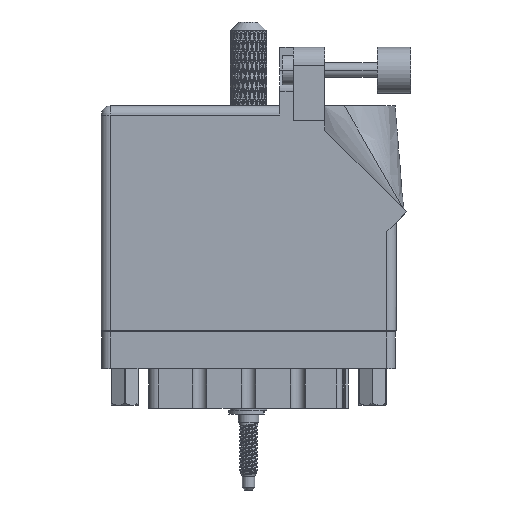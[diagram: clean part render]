
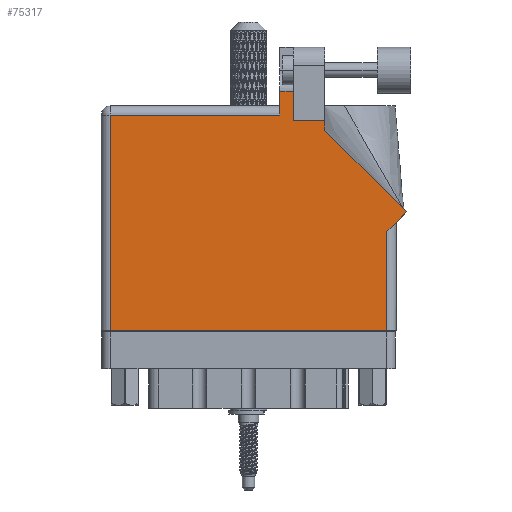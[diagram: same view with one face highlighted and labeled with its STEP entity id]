
A CAD part, front view. The second image highlights one B-rep face of the part: STEP entity #75317.
In plain terms, the highlighted face is planar.
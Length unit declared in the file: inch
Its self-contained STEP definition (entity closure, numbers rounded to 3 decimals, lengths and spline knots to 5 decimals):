
#374 = EDGE_CURVE ( 'NONE', #49870, #22491, #19610, .T. ) ;
#800 = VERTEX_POINT ( 'NONE', #60973 ) ;
#1143 = VECTOR ( 'NONE', #28978, 39.37008 ) ;
#1343 = CARTESIAN_POINT ( 'NONE',  ( 0.062, 0., 0. ) ) ;
#2345 = LINE ( 'NONE', #21454, #79653 ) ;
#4068 = CARTESIAN_POINT ( 'NONE',  ( 2.01, 0.737, 0. ) ) ;
#5318 = EDGE_CURVE ( 'NONE', #39383, #42970, #53773, .T. ) ;
#5324 = VECTOR ( 'NONE', #37915, 39.37008 ) ;
#5744 = EDGE_LOOP ( 'NONE', ( #24149, #11952, #10577, #45719, #68616, #12436, #71256, #103133, #88107, #72380, #15375 ) ) ;
#5793 = EDGE_CURVE ( 'NONE', #79085, #9011, #2345, .T. ) ;
#8879 = VECTOR ( 'NONE', #9280, 39.37008 ) ;
#9011 = VERTEX_POINT ( 'NONE', #25534 ) ;
#9280 = DIRECTION ( 'NONE',  ( -1., 0., 0. ) ) ;
#10577 = ORIENTED_EDGE ( 'NONE', *, *, #5793, .T. ) ;
#10686 = DIRECTION ( 'NONE',  ( 1., 0., 0. ) ) ;
#11869 = VECTOR ( 'NONE', #85549, 39.37008 ) ;
#11952 = ORIENTED_EDGE ( 'NONE', *, *, #102601, .T. ) ;
#12096 = CARTESIAN_POINT ( 'NONE',  ( 1.524, 1.36442, 0. ) ) ;
#12436 = ORIENTED_EDGE ( 'NONE', *, *, #32887, .T. ) ;
#14048 = DIRECTION ( 'NONE',  ( -1., 0., 0. ) ) ;
#15375 = ORIENTED_EDGE ( 'NONE', *, *, #78607, .T. ) ;
#15403 = EDGE_CURVE ( 'NONE', #61928, #29039, #55315, .T. ) ;
#19053 = CARTESIAN_POINT ( 'NONE',  ( 1.524, 1.43, 0. ) ) ;
#19610 = LINE ( 'NONE', #12096, #31677 ) ;
#21454 = CARTESIAN_POINT ( 'NONE',  ( 1.217, 1.53, 0. ) ) ;
#21537 = CARTESIAN_POINT ( 'NONE',  ( 1.311, 1.43, 0. ) ) ;
#22491 = VERTEX_POINT ( 'NONE', #109460 ) ;
#24149 = ORIENTED_EDGE ( 'NONE', *, *, #5318, .T. ) ;
#24652 = LINE ( 'NONE', #53649, #103189 ) ;
#25534 = CARTESIAN_POINT ( 'NONE',  ( 1.217, 1.468, 0. ) ) ;
#26724 = LINE ( 'NONE', #102984, #11869 ) ;
#27309 = EDGE_CURVE ( 'NONE', #29039, #800, #70169, .T. ) ;
#27651 = CARTESIAN_POINT ( 'NONE',  ( 0., 0., 0. ) ) ;
#28978 = DIRECTION ( 'NONE',  ( 0.707, 0.707, 0. ) ) ;
#29039 = VERTEX_POINT ( 'NONE', #96238 ) ;
#29055 = VERTEX_POINT ( 'NONE', #1343 ) ;
#30135 = CARTESIAN_POINT ( 'NONE',  ( 1.948, 0., 0. ) ) ;
#30700 = VECTOR ( 'NONE', #32224, 39.37008 ) ;
#31677 = VECTOR ( 'NONE', #89605, 39.37008 ) ;
#32224 = DIRECTION ( 'NONE',  ( 0., 1., 0. ) ) ;
#32887 = EDGE_CURVE ( 'NONE', #29055, #61928, #50562, .T. ) ;
#33662 = CARTESIAN_POINT ( 'NONE',  ( 0.062, 1.468, 0. ) ) ;
#37915 = DIRECTION ( 'NONE',  ( 0., 1., 0. ) ) ;
#38689 = EDGE_CURVE ( 'NONE', #46839, #29055, #26724, .T. ) ;
#39383 = VERTEX_POINT ( 'NONE', #21537 ) ;
#42509 = CARTESIAN_POINT ( 'NONE',  ( 1.948, 0.737, 0. ) ) ;
#42970 = VERTEX_POINT ( 'NONE', #43182 ) ;
#43058 = VECTOR ( 'NONE', #102209, 39.37008 ) ;
#43182 = CARTESIAN_POINT ( 'NONE',  ( 1.311, 1.6315, 0. ) ) ;
#45719 = ORIENTED_EDGE ( 'NONE', *, *, #107724, .T. ) ;
#46839 = VERTEX_POINT ( 'NONE', #33662 ) ;
#48945 = VECTOR ( 'NONE', #61003, 39.37008 ) ;
#49870 = VERTEX_POINT ( 'NONE', #84795 ) ;
#50562 = LINE ( 'NONE', #27651, #68102 ) ;
#52519 = EDGE_CURVE ( 'NONE', #800, #49870, #62511, .T. ) ;
#53649 = CARTESIAN_POINT ( 'NONE',  ( 1.64177, 1.6315, 0. ) ) ;
#53773 = LINE ( 'NONE', #83693, #30700 ) ;
#55315 = LINE ( 'NONE', #42509, #5324 ) ;
#57174 = CARTESIAN_POINT ( 'NONE',  ( 0., 1.53, 0. ) ) ;
#57375 = AXIS2_PLACEMENT_3D ( 'NONE', #57174, #91932, #14048 ) ;
#57418 = DIRECTION ( 'NONE',  ( 0., -1., 0. ) ) ;
#60973 = CARTESIAN_POINT ( 'NONE',  ( 2.08071, 0.80771, 0. ) ) ;
#61003 = DIRECTION ( 'NONE',  ( -0.707, 0.707, 0. ) ) ;
#61928 = VERTEX_POINT ( 'NONE', #30135 ) ;
#62511 = LINE ( 'NONE', #86646, #48945 ) ;
#66262 = CARTESIAN_POINT ( 'NONE',  ( 0., 1.468, 0. ) ) ;
#66988 = LINE ( 'NONE', #19053, #8879 ) ;
#68102 = VECTOR ( 'NONE', #10686, 39.37008 ) ;
#68616 = ORIENTED_EDGE ( 'NONE', *, *, #38689, .T. ) ;
#70169 = LINE ( 'NONE', #4068, #1143 ) ;
#70696 = DIRECTION ( 'NONE',  ( -1., 0., 0. ) ) ;
#71099 = CARTESIAN_POINT ( 'NONE',  ( 1.217, 1.6315, 0. ) ) ;
#71256 = ORIENTED_EDGE ( 'NONE', *, *, #15403, .T. ) ;
#72380 = ORIENTED_EDGE ( 'NONE', *, *, #374, .T. ) ;
#75317 = ADVANCED_FACE ( 'NONE', ( #77226 ), #101438, .F. ) ;
#77226 = FACE_OUTER_BOUND ( 'NONE', #5744, .T. ) ;
#78607 = EDGE_CURVE ( 'NONE', #22491, #39383, #66988, .T. ) ;
#79085 = VERTEX_POINT ( 'NONE', #71099 ) ;
#79653 = VECTOR ( 'NONE', #57418, 39.37008 ) ;
#83693 = CARTESIAN_POINT ( 'NONE',  ( 1.311, 1.43, 0. ) ) ;
#84795 = CARTESIAN_POINT ( 'NONE',  ( 1.524, 1.36442, 0. ) ) ;
#85549 = DIRECTION ( 'NONE',  ( 0., -1., 0. ) ) ;
#86646 = CARTESIAN_POINT ( 'NONE',  ( 2.08071, 0.80771, 0. ) ) ;
#88107 = ORIENTED_EDGE ( 'NONE', *, *, #52519, .T. ) ;
#89605 = DIRECTION ( 'NONE',  ( 0., 1., 0. ) ) ;
#91932 = DIRECTION ( 'NONE',  ( 0., 0., -1. ) ) ;
#96238 = CARTESIAN_POINT ( 'NONE',  ( 1.948, 0.675, 0. ) ) ;
#98543 = LINE ( 'NONE', #66262, #43058 ) ;
#101438 = PLANE ( 'NONE',  #57375 ) ;
#102209 = DIRECTION ( 'NONE',  ( -1., 0., 0. ) ) ;
#102601 = EDGE_CURVE ( 'NONE', #42970, #79085, #24652, .T. ) ;
#102984 = CARTESIAN_POINT ( 'NONE',  ( 0.062, 0., 0. ) ) ;
#103133 = ORIENTED_EDGE ( 'NONE', *, *, #27309, .T. ) ;
#103189 = VECTOR ( 'NONE', #70696, 39.37008 ) ;
#107724 = EDGE_CURVE ( 'NONE', #9011, #46839, #98543, .T. ) ;
#109460 = CARTESIAN_POINT ( 'NONE',  ( 1.524, 1.43, 0. ) ) ;
